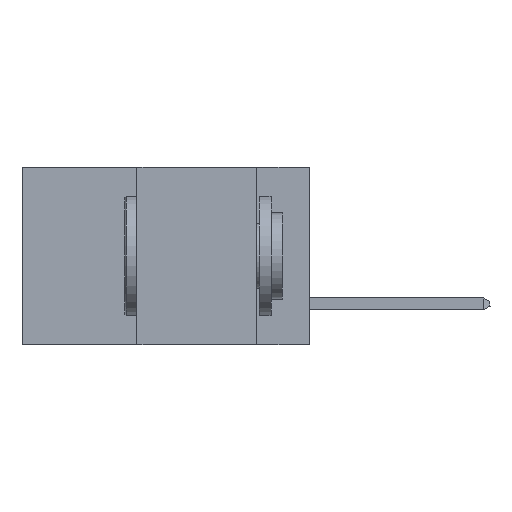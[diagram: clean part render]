
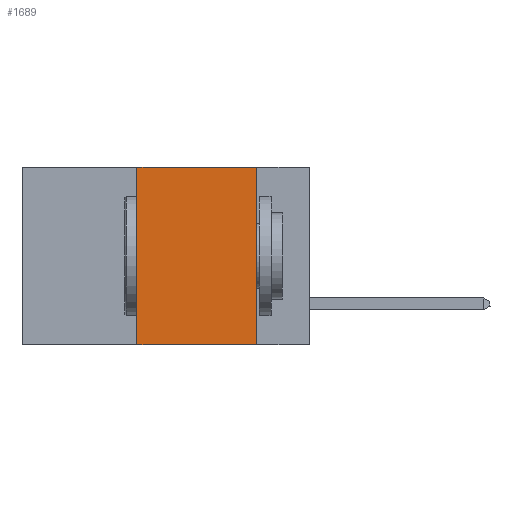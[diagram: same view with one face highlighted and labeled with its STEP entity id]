
A CAD part, left-side view. The second image highlights one B-rep face of the part: STEP entity #1689.
In plain terms, the highlighted planar face has unit normal (-1, 0, 0).
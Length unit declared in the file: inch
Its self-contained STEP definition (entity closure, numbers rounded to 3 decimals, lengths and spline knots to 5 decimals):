
#1689 = ADVANCED_FACE ( 'NONE', ( #16118 ), #5246, .F. ) ;
#1780 = LINE ( 'NONE', #4903, #38413 ) ;
#2532 = VERTEX_POINT ( 'NONE', #26346 ) ;
#2939 = ORIENTED_EDGE ( 'NONE', *, *, #23375, .F. ) ;
#4903 = CARTESIAN_POINT ( 'NONE',  ( 0., 0.6, -0.37 ) ) ;
#5246 = PLANE ( 'NONE',  #37540 ) ;
#8013 = LINE ( 'NONE', #31018, #40240 ) ;
#8647 = DIRECTION ( 'NONE',  ( 1., 0., 0. ) ) ;
#10740 = EDGE_CURVE ( 'NONE', #2532, #45842, #1780, .T. ) ;
#12793 = EDGE_CURVE ( 'NONE', #28733, #45842, #26581, .T. ) ;
#16118 = FACE_OUTER_BOUND ( 'NONE', #27981, .T. ) ;
#17859 = EDGE_CURVE ( 'NONE', #32524, #28733, #33560, .T. ) ;
#18509 = CARTESIAN_POINT ( 'NONE',  ( 0., 0.11, 0. ) ) ;
#19122 = VECTOR ( 'NONE', #32298, 39.37008 ) ;
#19295 = CARTESIAN_POINT ( 'NONE',  ( 0., 0.11, -0.37 ) ) ;
#19440 = DIRECTION ( 'NONE',  ( 0., 0., -1. ) ) ;
#20001 = DIRECTION ( 'NONE',  ( 0., 0., 1. ) ) ;
#20125 = CARTESIAN_POINT ( 'NONE',  ( 0., 0.36, 0. ) ) ;
#22650 = ORIENTED_EDGE ( 'NONE', *, *, #10740, .T. ) ;
#23375 = EDGE_CURVE ( 'NONE', #2532, #32524, #8013, .T. ) ;
#26346 = CARTESIAN_POINT ( 'NONE',  ( 0., 0.36, -0.37 ) ) ;
#26581 = LINE ( 'NONE', #40513, #39323 ) ;
#26838 = DIRECTION ( 'NONE',  ( 0., 0., -1. ) ) ;
#27981 = EDGE_LOOP ( 'NONE', ( #45406, #31962, #2939, #22650 ) ) ;
#28698 = CARTESIAN_POINT ( 'NONE',  ( 0., 0.6, 0. ) ) ;
#28733 = VERTEX_POINT ( 'NONE', #18509 ) ;
#31018 = CARTESIAN_POINT ( 'NONE',  ( 0., 0.36, 0. ) ) ;
#31962 = ORIENTED_EDGE ( 'NONE', *, *, #17859, .F. ) ;
#32298 = DIRECTION ( 'NONE',  ( 0., -1., 0. ) ) ;
#32524 = VERTEX_POINT ( 'NONE', #20125 ) ;
#33560 = LINE ( 'NONE', #28698, #19122 ) ;
#37540 = AXIS2_PLACEMENT_3D ( 'NONE', #41246, #8647, #19440 ) ;
#38413 = VECTOR ( 'NONE', #40734, 39.37008 ) ;
#39323 = VECTOR ( 'NONE', #26838, 39.37008 ) ;
#40240 = VECTOR ( 'NONE', #20001, 39.37008 ) ;
#40513 = CARTESIAN_POINT ( 'NONE',  ( 0., 0.11, 0. ) ) ;
#40734 = DIRECTION ( 'NONE',  ( 0., -1., 0. ) ) ;
#41246 = CARTESIAN_POINT ( 'NONE',  ( 0., 0.6, 0. ) ) ;
#45406 = ORIENTED_EDGE ( 'NONE', *, *, #12793, .F. ) ;
#45842 = VERTEX_POINT ( 'NONE', #19295 ) ;
